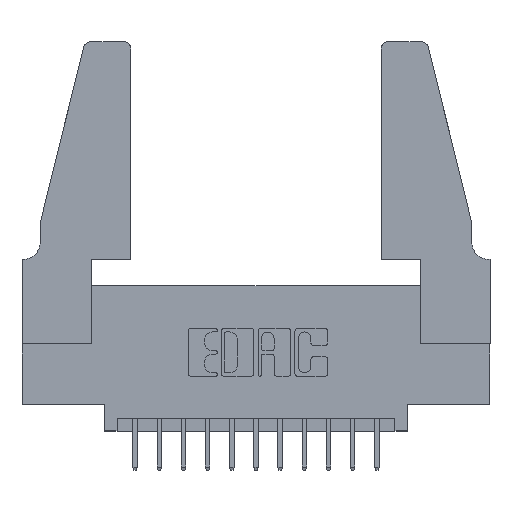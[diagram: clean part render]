
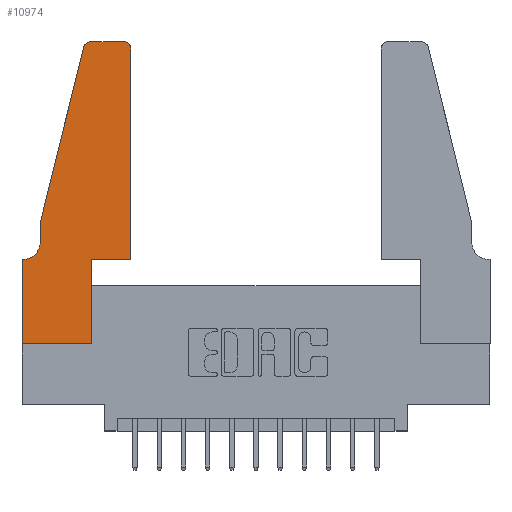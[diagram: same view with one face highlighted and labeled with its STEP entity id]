
A CAD part, top view. The second image highlights one B-rep face of the part: STEP entity #10974.
In plain terms, the highlighted planar face has unit normal (0, 0, 1).
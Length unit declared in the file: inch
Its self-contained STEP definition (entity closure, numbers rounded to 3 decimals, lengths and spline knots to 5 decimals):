
#18 = CARTESIAN_POINT ( 'NONE',  ( 0.2865, 0., 0.37 ) ) ;
#96 = DIRECTION ( 'NONE',  ( 0., 1., 0. ) ) ;
#178 = CARTESIAN_POINT ( 'NONE',  ( 0.4505, 0.35, 0.37 ) ) ;
#183 = VERTEX_POINT ( 'NONE', #3046 ) ;
#346 = VERTEX_POINT ( 'NONE', #7305 ) ;
#524 = EDGE_CURVE ( 'NONE', #12240, #11991, #2663, .T. ) ;
#626 = LINE ( 'NONE', #2979, #2649 ) ;
#693 = DIRECTION ( 'NONE',  ( -1., 0., 0. ) ) ;
#763 = VECTOR ( 'NONE', #10103, 39.37008 ) ;
#872 = EDGE_CURVE ( 'NONE', #346, #8353, #626, .T. ) ;
#1239 = DIRECTION ( 'NONE',  ( 1., 0., 0. ) ) ;
#1296 = EDGE_CURVE ( 'NONE', #5461, #346, #9083, .T. ) ;
#1331 = DIRECTION ( 'NONE',  ( 1., 0., 0. ) ) ;
#1523 = CARTESIAN_POINT ( 'NONE',  ( 0., 0.35, 0.37 ) ) ;
#2121 = VECTOR ( 'NONE', #6435, 39.37008 ) ;
#2186 = ORIENTED_EDGE ( 'NONE', *, *, #5428, .T. ) ;
#2207 = VECTOR ( 'NONE', #8488, 39.37008 ) ;
#2540 = DIRECTION ( 'NONE',  ( 1., 0., 0. ) ) ;
#2649 = VECTOR ( 'NONE', #693, 39.37008 ) ;
#2663 = CIRCLE ( 'NONE', #14041, 0.03 ) ;
#2979 = CARTESIAN_POINT ( 'NONE',  ( 0.0755, 0.35, 0.37 ) ) ;
#2980 = CARTESIAN_POINT ( 'NONE',  ( 0., 0.35, 0.37 ) ) ;
#3046 = CARTESIAN_POINT ( 'NONE',  ( 0., 0., 0.37 ) ) ;
#3092 = CARTESIAN_POINT ( 'NONE',  ( 0.0755, 0.5, 0.37 ) ) ;
#3094 = ORIENTED_EDGE ( 'NONE', *, *, #1296, .T. ) ;
#3238 = LINE ( 'NONE', #14479, #2121 ) ;
#3424 = EDGE_CURVE ( 'NONE', #9071, #5461, #5564, .T. ) ;
#3445 = CARTESIAN_POINT ( 'NONE',  ( 0.4205, 1.25, 0.37 ) ) ;
#3639 = CARTESIAN_POINT ( 'NONE',  ( 0.2865, 0.35, 0.37 ) ) ;
#3756 = DIRECTION ( 'NONE',  ( 0., -1., 0. ) ) ;
#3858 = VECTOR ( 'NONE', #1239, 39.37008 ) ;
#3862 = ORIENTED_EDGE ( 'NONE', *, *, #10358, .T. ) ;
#5306 = VERTEX_POINT ( 'NONE', #18 ) ;
#5428 = EDGE_CURVE ( 'NONE', #5306, #9193, #15053, .T. ) ;
#5439 = CARTESIAN_POINT ( 'NONE',  ( 0.25487, 1.22718, 0.37 ) ) ;
#5461 = VERTEX_POINT ( 'NONE', #7216 ) ;
#5564 = LINE ( 'NONE', #8389, #9221 ) ;
#5610 = ORIENTED_EDGE ( 'NONE', *, *, #872, .T. ) ;
#5627 = CARTESIAN_POINT ( 'NONE',  ( 0.4505, 0.35, 0.37 ) ) ;
#5933 = AXIS2_PLACEMENT_3D ( 'NONE', #2980, #6906, #8234 ) ;
#6093 = EDGE_CURVE ( 'NONE', #9193, #9340, #10454, .T. ) ;
#6435 = DIRECTION ( 'NONE',  ( -1., 0., 0. ) ) ;
#6740 = EDGE_CURVE ( 'NONE', #10443, #8901, #13354, .T. ) ;
#6864 = LINE ( 'NONE', #3092, #12316 ) ;
#6881 = AXIS2_PLACEMENT_3D ( 'NONE', #7280, #13046, #1331 ) ;
#6906 = DIRECTION ( 'NONE',  ( 0., 0., 1. ) ) ;
#7165 = CARTESIAN_POINT ( 'NONE',  ( 0.2865, 0.35, 0.37 ) ) ;
#7216 = CARTESIAN_POINT ( 'NONE',  ( 0.0755, 0.42, 0.37 ) ) ;
#7280 = CARTESIAN_POINT ( 'NONE',  ( 0.284, 1.22, 0.37 ) ) ;
#7305 = CARTESIAN_POINT ( 'NONE',  ( 0.0055, 0.35, 0.37 ) ) ;
#7809 = DIRECTION ( 'NONE',  ( -1., 0., 0. ) ) ;
#7813 = CARTESIAN_POINT ( 'NONE',  ( 0.4205, 1.22, 0.37 ) ) ;
#8003 = AXIS2_PLACEMENT_3D ( 'NONE', #11268, #11116, #7809 ) ;
#8053 = EDGE_CURVE ( 'NONE', #11991, #10443, #3238, .T. ) ;
#8234 = DIRECTION ( 'NONE',  ( 1., 0., 0. ) ) ;
#8353 = VERTEX_POINT ( 'NONE', #1523 ) ;
#8389 = CARTESIAN_POINT ( 'NONE',  ( 0.0755, 0.5, 0.37 ) ) ;
#8488 = DIRECTION ( 'NONE',  ( 0., 1., 0. ) ) ;
#8901 = VERTEX_POINT ( 'NONE', #5439 ) ;
#9041 = FACE_OUTER_BOUND ( 'NONE', #9559, .T. ) ;
#9071 = VERTEX_POINT ( 'NONE', #11255 ) ;
#9083 = CIRCLE ( 'NONE', #8003, 0.07 ) ;
#9193 = VERTEX_POINT ( 'NONE', #3639 ) ;
#9221 = VECTOR ( 'NONE', #3756, 39.37008 ) ;
#9230 = ORIENTED_EDGE ( 'NONE', *, *, #524, .T. ) ;
#9340 = VERTEX_POINT ( 'NONE', #15023 ) ;
#9365 = DIRECTION ( 'NONE',  ( -0.239, -0.971, 0. ) ) ;
#9520 = EDGE_CURVE ( 'NONE', #8353, #183, #9796, .T. ) ;
#9559 = EDGE_LOOP ( 'NONE', ( #13239, #14262, #3862, #12603, #3094, #5610, #12186, #15003, #2186, #13139, #15067, #9230 ) ) ;
#9796 = LINE ( 'NONE', #11211, #763 ) ;
#10103 = DIRECTION ( 'NONE',  ( 0., -1., 0. ) ) ;
#10263 = DIRECTION ( 'NONE',  ( 1., 0., 0. ) ) ;
#10354 = DIRECTION ( 'NONE',  ( 0., 0., 1. ) ) ;
#10358 = EDGE_CURVE ( 'NONE', #8901, #9071, #6864, .T. ) ;
#10443 = VERTEX_POINT ( 'NONE', #13129 ) ;
#10454 = LINE ( 'NONE', #178, #11168 ) ;
#10659 = EDGE_CURVE ( 'NONE', #9340, #12240, #12862, .T. ) ;
#10841 = LINE ( 'NONE', #14261, #3858 ) ;
#10974 = ADVANCED_FACE ( 'NONE', ( #9041 ), #12712, .T. ) ;
#11116 = DIRECTION ( 'NONE',  ( 0., 0., -1. ) ) ;
#11168 = VECTOR ( 'NONE', #2540, 39.37008 ) ;
#11211 = CARTESIAN_POINT ( 'NONE',  ( 0., 0., 0.37 ) ) ;
#11255 = CARTESIAN_POINT ( 'NONE',  ( 0.0755, 0.5, 0.37 ) ) ;
#11268 = CARTESIAN_POINT ( 'NONE',  ( 0.0055, 0.42, 0.37 ) ) ;
#11689 = EDGE_CURVE ( 'NONE', #183, #5306, #10841, .T. ) ;
#11991 = VERTEX_POINT ( 'NONE', #3445 ) ;
#12186 = ORIENTED_EDGE ( 'NONE', *, *, #9520, .T. ) ;
#12240 = VERTEX_POINT ( 'NONE', #15140 ) ;
#12291 = VECTOR ( 'NONE', #96, 39.37008 ) ;
#12316 = VECTOR ( 'NONE', #9365, 39.37008 ) ;
#12603 = ORIENTED_EDGE ( 'NONE', *, *, #3424, .T. ) ;
#12712 = PLANE ( 'NONE',  #5933 ) ;
#12862 = LINE ( 'NONE', #5627, #12291 ) ;
#13046 = DIRECTION ( 'NONE',  ( 0., 0., 1. ) ) ;
#13129 = CARTESIAN_POINT ( 'NONE',  ( 0.284, 1.25, 0.37 ) ) ;
#13139 = ORIENTED_EDGE ( 'NONE', *, *, #6093, .T. ) ;
#13239 = ORIENTED_EDGE ( 'NONE', *, *, #8053, .T. ) ;
#13354 = CIRCLE ( 'NONE', #6881, 0.03 ) ;
#14041 = AXIS2_PLACEMENT_3D ( 'NONE', #7813, #10354, #10263 ) ;
#14261 = CARTESIAN_POINT ( 'NONE',  ( 0., 0., 0.37 ) ) ;
#14262 = ORIENTED_EDGE ( 'NONE', *, *, #6740, .T. ) ;
#14479 = CARTESIAN_POINT ( 'NONE',  ( 0.2605, 1.25, 0.37 ) ) ;
#15003 = ORIENTED_EDGE ( 'NONE', *, *, #11689, .T. ) ;
#15023 = CARTESIAN_POINT ( 'NONE',  ( 0.4505, 0.35, 0.37 ) ) ;
#15053 = LINE ( 'NONE', #7165, #2207 ) ;
#15067 = ORIENTED_EDGE ( 'NONE', *, *, #10659, .T. ) ;
#15140 = CARTESIAN_POINT ( 'NONE',  ( 0.4505, 1.22, 0.37 ) ) ;
